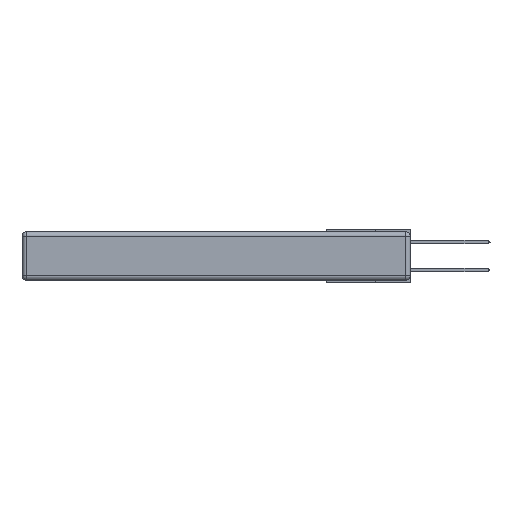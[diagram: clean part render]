
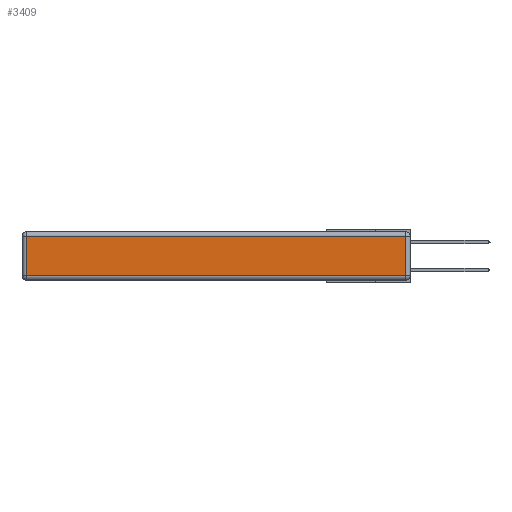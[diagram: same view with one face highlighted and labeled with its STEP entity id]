
A CAD part, left-side view. The second image highlights one B-rep face of the part: STEP entity #3409.
In plain terms, the highlighted planar face has unit normal (-1, 0, 0).
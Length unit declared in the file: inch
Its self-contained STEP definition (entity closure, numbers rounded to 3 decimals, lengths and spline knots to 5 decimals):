
#1129 = ORIENTED_EDGE ( 'NONE', *, *, #9588, .T. ) ;
#1264 = VECTOR ( 'NONE', #1517, 39.37008 ) ;
#1517 = DIRECTION ( 'NONE',  ( 0., 0., -1. ) ) ;
#2973 = LINE ( 'NONE', #25332, #7422 ) ;
#3409 = ADVANCED_FACE ( 'NONE', ( #26704 ), #3891, .T. ) ;
#3891 = PLANE ( 'NONE',  #24088 ) ;
#3897 = LINE ( 'NONE', #8123, #26437 ) ;
#3962 = DIRECTION ( 'NONE',  ( 0., 0., 1. ) ) ;
#4664 = CARTESIAN_POINT ( 'NONE',  ( 0., 2.72, -0.313 ) ) ;
#5216 = VERTEX_POINT ( 'NONE', #4664 ) ;
#5285 = ORIENTED_EDGE ( 'NONE', *, *, #14097, .T. ) ;
#5646 = DIRECTION ( 'NONE',  ( 0., 1., 0. ) ) ;
#5801 = DIRECTION ( 'NONE',  ( -1., 0., 0. ) ) ;
#7422 = VECTOR ( 'NONE', #5646, 39.37008 ) ;
#7546 = LINE ( 'NONE', #23559, #8903 ) ;
#7747 = VERTEX_POINT ( 'NONE', #21822 ) ;
#8123 = CARTESIAN_POINT ( 'NONE',  ( 0., 0., -0.313 ) ) ;
#8903 = VECTOR ( 'NONE', #3962, 39.37008 ) ;
#9588 = EDGE_CURVE ( 'NONE', #5216, #7747, #3897, .T. ) ;
#14097 = EDGE_CURVE ( 'NONE', #16336, #17912, #2973, .T. ) ;
#14515 = EDGE_CURVE ( 'NONE', #17912, #5216, #28218, .T. ) ;
#16336 = VERTEX_POINT ( 'NONE', #18879 ) ;
#17048 = DIRECTION ( 'NONE',  ( 0., -1., 0. ) ) ;
#17912 = VERTEX_POINT ( 'NONE', #27048 ) ;
#18879 = CARTESIAN_POINT ( 'NONE',  ( 0., 0.03, -0.03 ) ) ;
#21822 = CARTESIAN_POINT ( 'NONE',  ( 0., 0.03, -0.313 ) ) ;
#23426 = ORIENTED_EDGE ( 'NONE', *, *, #14515, .T. ) ;
#23559 = CARTESIAN_POINT ( 'NONE',  ( 0., 0.03, -0.343 ) ) ;
#24088 = AXIS2_PLACEMENT_3D ( 'NONE', #27563, #5801, #25495 ) ;
#24282 = EDGE_LOOP ( 'NONE', ( #1129, #24636, #5285, #23426 ) ) ;
#24636 = ORIENTED_EDGE ( 'NONE', *, *, #27416, .T. ) ;
#25332 = CARTESIAN_POINT ( 'NONE',  ( 0., 2.75, -0.03 ) ) ;
#25495 = DIRECTION ( 'NONE',  ( 0., 0., 1. ) ) ;
#26437 = VECTOR ( 'NONE', #17048, 39.37008 ) ;
#26704 = FACE_OUTER_BOUND ( 'NONE', #24282, .T. ) ;
#27048 = CARTESIAN_POINT ( 'NONE',  ( 0., 2.72, -0.03 ) ) ;
#27416 = EDGE_CURVE ( 'NONE', #7747, #16336, #7546, .T. ) ;
#27563 = CARTESIAN_POINT ( 'NONE',  ( 0., 0., -0.343 ) ) ;
#27645 = CARTESIAN_POINT ( 'NONE',  ( 0., 2.72, -0.343 ) ) ;
#28218 = LINE ( 'NONE', #27645, #1264 ) ;
